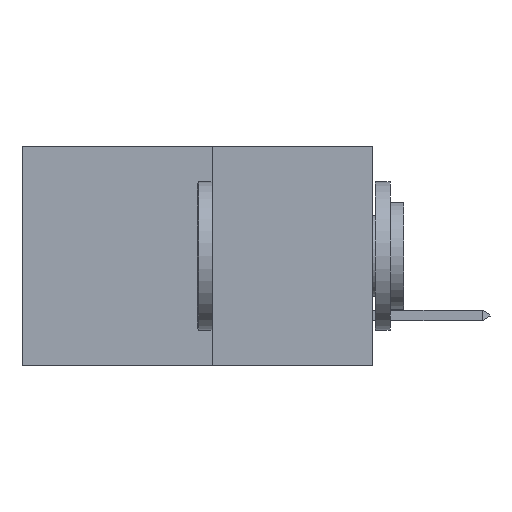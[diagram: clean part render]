
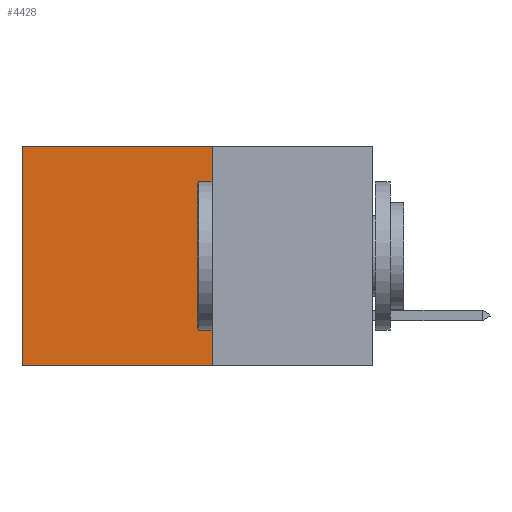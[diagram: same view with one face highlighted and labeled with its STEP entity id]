
A CAD part, left-side view. The second image highlights one B-rep face of the part: STEP entity #4428.
In plain terms, the highlighted planar face has unit normal (-1, 0, 0).
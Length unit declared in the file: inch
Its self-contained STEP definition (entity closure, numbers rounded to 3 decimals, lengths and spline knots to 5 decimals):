
#2 = ORIENTED_EDGE ( 'NONE', *, *, #12077, .F. ) ;
#10 = EDGE_CURVE ( 'NONE', #7920, #2976, #10913, .T. ) ;
#550 = VERTEX_POINT ( 'NONE', #4423 ) ;
#694 = DIRECTION ( 'NONE',  ( 1., 0., 0. ) ) ;
#1130 = CARTESIAN_POINT ( 'NONE',  ( 0.277, 0.59, -0.37 ) ) ;
#1868 = LINE ( 'NONE', #1130, #7384 ) ;
#2385 = ORIENTED_EDGE ( 'NONE', *, *, #12639, .T. ) ;
#2614 = DIRECTION ( 'NONE',  ( 0., 1., 0. ) ) ;
#2976 = VERTEX_POINT ( 'NONE', #4033 ) ;
#3981 = FACE_OUTER_BOUND ( 'NONE', #13984, .T. ) ;
#4033 = CARTESIAN_POINT ( 'NONE',  ( 0.277, 0.27, -0.37 ) ) ;
#4105 = AXIS2_PLACEMENT_3D ( 'NONE', #7864, #694, #8945 ) ;
#4423 = CARTESIAN_POINT ( 'NONE',  ( 0.277, 0.59, -0.37 ) ) ;
#4428 = ADVANCED_FACE ( 'NONE', ( #3981 ), #5555, .F. ) ;
#4555 = DIRECTION ( 'NONE',  ( 0., 1., 0. ) ) ;
#5555 = PLANE ( 'NONE',  #4105 ) ;
#5699 = EDGE_CURVE ( 'NONE', #10180, #550, #1868, .T. ) ;
#5875 = ORIENTED_EDGE ( 'NONE', *, *, #5699, .T. ) ;
#6153 = LINE ( 'NONE', #10488, #14632 ) ;
#7384 = VECTOR ( 'NONE', #8207, 39.37008 ) ;
#7864 = CARTESIAN_POINT ( 'NONE',  ( 0.277, 0.27, -0.37 ) ) ;
#7920 = VERTEX_POINT ( 'NONE', #10716 ) ;
#8207 = DIRECTION ( 'NONE',  ( 0., 0., -1. ) ) ;
#8665 = CARTESIAN_POINT ( 'NONE',  ( 0.277, 0.59, 0. ) ) ;
#8819 = VECTOR ( 'NONE', #4555, 39.37008 ) ;
#8945 = DIRECTION ( 'NONE',  ( 0., 0., -1. ) ) ;
#10180 = VERTEX_POINT ( 'NONE', #8665 ) ;
#10488 = CARTESIAN_POINT ( 'NONE',  ( 0.277, 0.27, 0. ) ) ;
#10581 = VECTOR ( 'NONE', #13767, 39.37008 ) ;
#10716 = CARTESIAN_POINT ( 'NONE',  ( 0.277, 0.27, 0. ) ) ;
#10913 = LINE ( 'NONE', #13187, #10581 ) ;
#11934 = LINE ( 'NONE', #12209, #8819 ) ;
#12077 = EDGE_CURVE ( 'NONE', #2976, #550, #11934, .T. ) ;
#12209 = CARTESIAN_POINT ( 'NONE',  ( 0.277, 0.27, -0.37 ) ) ;
#12639 = EDGE_CURVE ( 'NONE', #7920, #10180, #6153, .T. ) ;
#13187 = CARTESIAN_POINT ( 'NONE',  ( 0.277, 0.27, -0.37 ) ) ;
#13559 = ORIENTED_EDGE ( 'NONE', *, *, #10, .F. ) ;
#13767 = DIRECTION ( 'NONE',  ( 0., 0., -1. ) ) ;
#13984 = EDGE_LOOP ( 'NONE', ( #5875, #2, #13559, #2385 ) ) ;
#14632 = VECTOR ( 'NONE', #2614, 39.37008 ) ;
